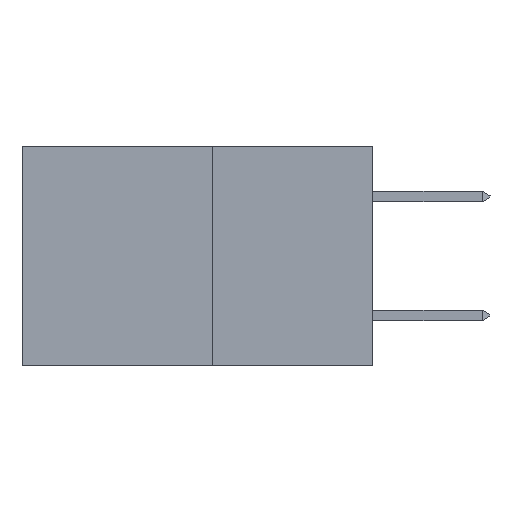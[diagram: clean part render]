
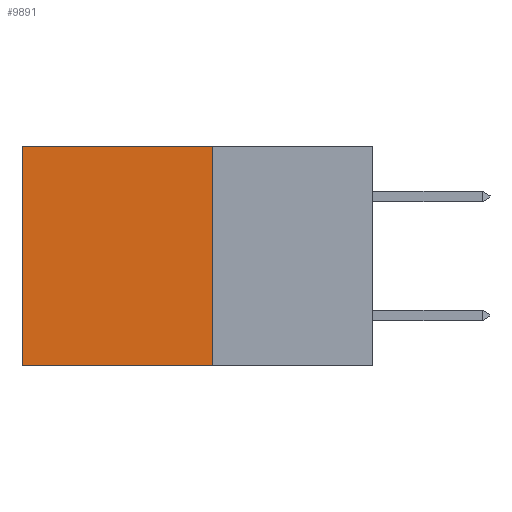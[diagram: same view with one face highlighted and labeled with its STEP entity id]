
A CAD part, left-side view. The second image highlights one B-rep face of the part: STEP entity #9891.
In plain terms, the highlighted planar face has unit normal (-1, 0, 0).
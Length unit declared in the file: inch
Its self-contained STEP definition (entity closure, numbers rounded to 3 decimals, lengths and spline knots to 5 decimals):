
#1174 = LINE ( 'NONE', #13059, #7637 ) ;
#1412 = EDGE_CURVE ( 'NONE', #23630, #32226, #3902, .T. ) ;
#2102 = CARTESIAN_POINT ( 'NONE',  ( 0.277, 0.59, 0. ) ) ;
#2712 = VECTOR ( 'NONE', #11475, 39.37008 ) ;
#3902 = LINE ( 'NONE', #7139, #24815 ) ;
#4066 = VERTEX_POINT ( 'NONE', #26135 ) ;
#4539 = EDGE_CURVE ( 'NONE', #32226, #22339, #30973, .T. ) ;
#4590 = DIRECTION ( 'NONE',  ( 1., 0., 0. ) ) ;
#7139 = CARTESIAN_POINT ( 'NONE',  ( 0.277, 0.27, 0. ) ) ;
#7637 = VECTOR ( 'NONE', #15772, 39.37008 ) ;
#8759 = EDGE_CURVE ( 'NONE', #4066, #22339, #31733, .T. ) ;
#9407 = DIRECTION ( 'NONE',  ( 0., 0., -1. ) ) ;
#9534 = FACE_OUTER_BOUND ( 'NONE', #11763, .T. ) ;
#9891 = ADVANCED_FACE ( 'NONE', ( #9534 ), #34444, .F. ) ;
#11350 = ORIENTED_EDGE ( 'NONE', *, *, #1412, .T. ) ;
#11475 = DIRECTION ( 'NONE',  ( 0., 1., 0. ) ) ;
#11763 = EDGE_LOOP ( 'NONE', ( #32055, #17944, #27088, #11350 ) ) ;
#13059 = CARTESIAN_POINT ( 'NONE',  ( 0.277, 0.27, -0.37 ) ) ;
#15401 = AXIS2_PLACEMENT_3D ( 'NONE', #20871, #4590, #24131 ) ;
#15520 = CARTESIAN_POINT ( 'NONE',  ( 0.277, 0.59, -0.37 ) ) ;
#15772 = DIRECTION ( 'NONE',  ( 0., 0., -1. ) ) ;
#17944 = ORIENTED_EDGE ( 'NONE', *, *, #8759, .F. ) ;
#18996 = DIRECTION ( 'NONE',  ( 0., 1., 0. ) ) ;
#19727 = EDGE_CURVE ( 'NONE', #23630, #4066, #1174, .T. ) ;
#20871 = CARTESIAN_POINT ( 'NONE',  ( 0.277, 0.27, -0.37 ) ) ;
#20956 = CARTESIAN_POINT ( 'NONE',  ( 0.277, 0.59, -0.37 ) ) ;
#22241 = CARTESIAN_POINT ( 'NONE',  ( 0.277, 0.27, -0.37 ) ) ;
#22339 = VERTEX_POINT ( 'NONE', #20956 ) ;
#23630 = VERTEX_POINT ( 'NONE', #35099 ) ;
#23718 = VECTOR ( 'NONE', #9407, 39.37008 ) ;
#24131 = DIRECTION ( 'NONE',  ( 0., 0., -1. ) ) ;
#24815 = VECTOR ( 'NONE', #18996, 39.37008 ) ;
#26135 = CARTESIAN_POINT ( 'NONE',  ( 0.277, 0.27, -0.37 ) ) ;
#27088 = ORIENTED_EDGE ( 'NONE', *, *, #19727, .F. ) ;
#30973 = LINE ( 'NONE', #15520, #23718 ) ;
#31733 = LINE ( 'NONE', #22241, #2712 ) ;
#32055 = ORIENTED_EDGE ( 'NONE', *, *, #4539, .T. ) ;
#32226 = VERTEX_POINT ( 'NONE', #2102 ) ;
#34444 = PLANE ( 'NONE',  #15401 ) ;
#35099 = CARTESIAN_POINT ( 'NONE',  ( 0.277, 0.27, 0. ) ) ;
